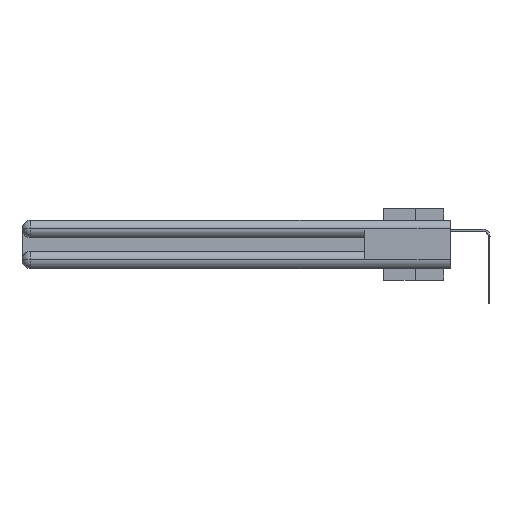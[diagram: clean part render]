
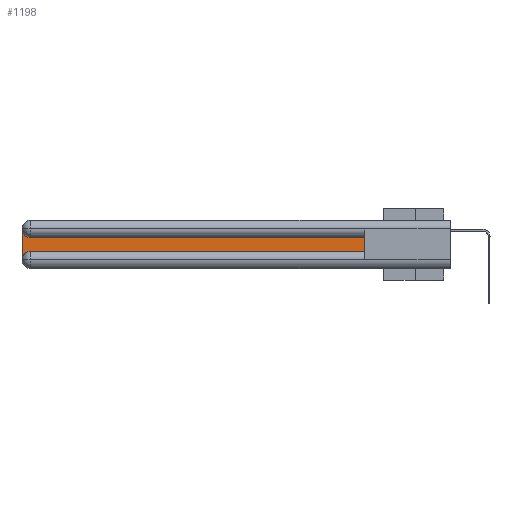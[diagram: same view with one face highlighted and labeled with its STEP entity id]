
A CAD part, left-side view. The second image highlights one B-rep face of the part: STEP entity #1198.
In plain terms, the highlighted planar face has unit normal (-1, 0, 0).
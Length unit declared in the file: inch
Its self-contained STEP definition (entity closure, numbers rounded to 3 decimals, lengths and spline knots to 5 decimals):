
#87 = AXIS2_PLACEMENT_3D ( 'NONE', #526, #22148, #10367 ) ;
#526 = CARTESIAN_POINT ( 'NONE',  ( 0.075, 2.94, -0.2775 ) ) ;
#712 = DIRECTION ( 'NONE',  ( 0., 1., 0. ) ) ;
#1198 = ADVANCED_FACE ( 'NONE', ( #4125 ), #17074, .F. ) ;
#1596 = AXIS2_PLACEMENT_3D ( 'NONE', #20089, #15426, #29860 ) ;
#1599 = CARTESIAN_POINT ( 'NONE',  ( 0.075, 2.94, -0.1225 ) ) ;
#2436 = LINE ( 'NONE', #26054, #6981 ) ;
#2669 = CARTESIAN_POINT ( 'NONE',  ( 0.075, 3., -0.1225 ) ) ;
#3528 = EDGE_CURVE ( 'NONE', #16200, #19071, #2436, .T. ) ;
#4125 = FACE_OUTER_BOUND ( 'NONE', #22822, .T. ) ;
#4235 = DIRECTION ( 'NONE',  ( 0., 0., -1. ) ) ;
#4481 = VECTOR ( 'NONE', #23672, 39.37008 ) ;
#6981 = VECTOR ( 'NONE', #4235, 39.37008 ) ;
#7850 = DIRECTION ( 'NONE',  ( 0., 0., -1. ) ) ;
#8756 = AXIS2_PLACEMENT_3D ( 'NONE', #2669, #27152, #7850 ) ;
#9398 = VERTEX_POINT ( 'NONE', #19535 ) ;
#10205 = ORIENTED_EDGE ( 'NONE', *, *, #30619, .T. ) ;
#10367 = DIRECTION ( 'NONE',  ( 0., 0., -1. ) ) ;
#11111 = ORIENTED_EDGE ( 'NONE', *, *, #17958, .T. ) ;
#12698 = VECTOR ( 'NONE', #17408, 39.37008 ) ;
#12976 = CARTESIAN_POINT ( 'NONE',  ( 0.075, 0.6, -0.1225 ) ) ;
#13554 = VERTEX_POINT ( 'NONE', #28456 ) ;
#13974 = CARTESIAN_POINT ( 'NONE',  ( 0.075, 0.6, -0.1225 ) ) ;
#14146 = LINE ( 'NONE', #12976, #28945 ) ;
#15426 = DIRECTION ( 'NONE',  ( 1., 0., 0. ) ) ;
#15738 = CARTESIAN_POINT ( 'NONE',  ( 0.075, 3., -0.2775 ) ) ;
#16200 = VERTEX_POINT ( 'NONE', #26292 ) ;
#16244 = CARTESIAN_POINT ( 'NONE',  ( 0.075, 0.6, -0.2175 ) ) ;
#16897 = LINE ( 'NONE', #29183, #12698 ) ;
#17074 = PLANE ( 'NONE',  #8756 ) ;
#17408 = DIRECTION ( 'NONE',  ( 0., -1., 0. ) ) ;
#17958 = EDGE_CURVE ( 'NONE', #9398, #28354, #24178, .T. ) ;
#18205 = EDGE_CURVE ( 'NONE', #19071, #13554, #19979, .T. ) ;
#19071 = VERTEX_POINT ( 'NONE', #15738 ) ;
#19535 = CARTESIAN_POINT ( 'NONE',  ( 0.075, 0.6, -0.2175 ) ) ;
#19979 = CIRCLE ( 'NONE', #87, 0.06 ) ;
#20089 = CARTESIAN_POINT ( 'NONE',  ( 0.075, 2.94, -0.0625 ) ) ;
#21319 = ORIENTED_EDGE ( 'NONE', *, *, #3528, .T. ) ;
#22148 = DIRECTION ( 'NONE',  ( 1., 0., 0. ) ) ;
#22822 = EDGE_LOOP ( 'NONE', ( #26148, #10205, #21319, #28078, #27501, #11111 ) ) ;
#23672 = DIRECTION ( 'NONE',  ( 0., 0., 1. ) ) ;
#24178 = LINE ( 'NONE', #16244, #4481 ) ;
#24253 = CIRCLE ( 'NONE', #1596, 0.06 ) ;
#26054 = CARTESIAN_POINT ( 'NONE',  ( 0.075, 3., -0.2175 ) ) ;
#26148 = ORIENTED_EDGE ( 'NONE', *, *, #28785, .T. ) ;
#26292 = CARTESIAN_POINT ( 'NONE',  ( 0.075, 3., -0.0625 ) ) ;
#27152 = DIRECTION ( 'NONE',  ( 1., 0., 0. ) ) ;
#27501 = ORIENTED_EDGE ( 'NONE', *, *, #27946, .T. ) ;
#27946 = EDGE_CURVE ( 'NONE', #13554, #9398, #16897, .T. ) ;
#28078 = ORIENTED_EDGE ( 'NONE', *, *, #18205, .T. ) ;
#28354 = VERTEX_POINT ( 'NONE', #13974 ) ;
#28456 = CARTESIAN_POINT ( 'NONE',  ( 0.075, 2.94, -0.2175 ) ) ;
#28785 = EDGE_CURVE ( 'NONE', #28354, #30264, #14146, .T. ) ;
#28945 = VECTOR ( 'NONE', #712, 39.37008 ) ;
#29183 = CARTESIAN_POINT ( 'NONE',  ( 0.075, 0.6, -0.2175 ) ) ;
#29860 = DIRECTION ( 'NONE',  ( 0., 0., -1. ) ) ;
#30264 = VERTEX_POINT ( 'NONE', #1599 ) ;
#30619 = EDGE_CURVE ( 'NONE', #30264, #16200, #24253, .T. ) ;
